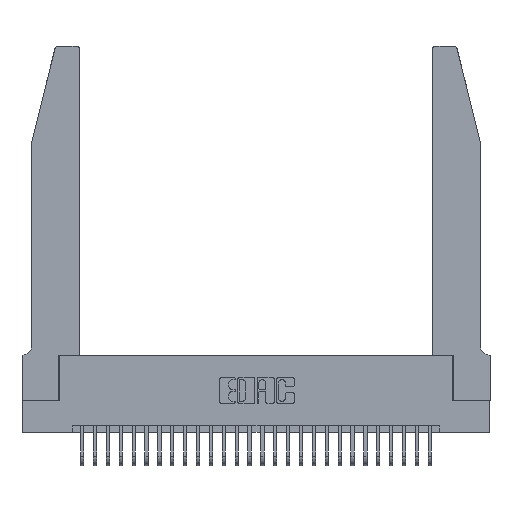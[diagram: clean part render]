
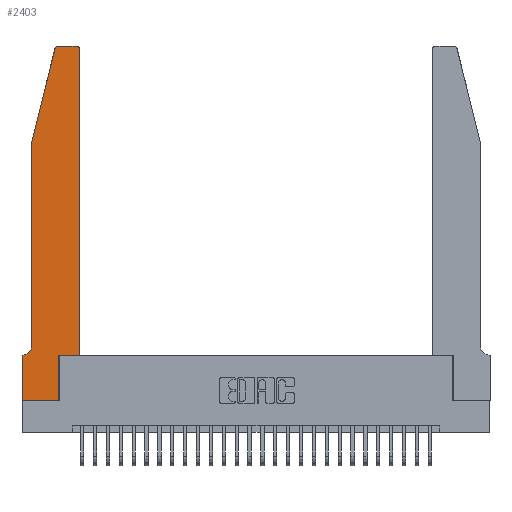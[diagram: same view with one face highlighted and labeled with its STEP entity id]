
A CAD part, top view. The second image highlights one B-rep face of the part: STEP entity #2403.
In plain terms, the highlighted planar face has unit normal (0, 0, 1).
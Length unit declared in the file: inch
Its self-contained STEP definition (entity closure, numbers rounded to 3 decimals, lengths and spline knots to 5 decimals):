
#251 = VECTOR ( 'NONE', #26868, 39.37008 ) ;
#269 = ORIENTED_EDGE ( 'NONE', *, *, #28386, .T. ) ;
#746 = LINE ( 'NONE', #19874, #24188 ) ;
#1655 = ORIENTED_EDGE ( 'NONE', *, *, #4228, .T. ) ;
#1901 = LINE ( 'NONE', #18953, #28568 ) ;
#1916 = CARTESIAN_POINT ( 'NONE',  ( 0., 0.35, 0.37 ) ) ;
#2403 = ADVANCED_FACE ( 'NONE', ( #9724 ), #2414, .T. ) ;
#2414 = PLANE ( 'NONE',  #26581 ) ;
#2914 = DIRECTION ( 'NONE',  ( -1., 0., 0. ) ) ;
#2936 = DIRECTION ( 'NONE',  ( 1., 0., 0. ) ) ;
#3030 = CIRCLE ( 'NONE', #27267, 0.07 ) ;
#3204 = VECTOR ( 'NONE', #20002, 39.37008 ) ;
#3740 = DIRECTION ( 'NONE',  ( 0., -1., 0. ) ) ;
#3985 = VECTOR ( 'NONE', #7193, 39.37008 ) ;
#4228 = EDGE_CURVE ( 'NONE', #15981, #23874, #29718, .T. ) ;
#4891 = LINE ( 'NONE', #24544, #8936 ) ;
#5684 = EDGE_CURVE ( 'NONE', #23874, #6973, #746, .T. ) ;
#6844 = LINE ( 'NONE', #10488, #251 ) ;
#6973 = VERTEX_POINT ( 'NONE', #12463 ) ;
#7193 = DIRECTION ( 'NONE',  ( 0., -1., 0. ) ) ;
#7324 = CARTESIAN_POINT ( 'NONE',  ( 0.4505, 2.72, 0.37 ) ) ;
#7369 = AXIS2_PLACEMENT_3D ( 'NONE', #26047, #12041, #28378 ) ;
#7442 = EDGE_CURVE ( 'NONE', #20556, #12438, #6844, .T. ) ;
#8609 = DIRECTION ( 'NONE',  ( -1., 0., 0. ) ) ;
#8773 = DIRECTION ( 'NONE',  ( 0., 1., 0. ) ) ;
#8936 = VECTOR ( 'NONE', #12594, 39.37008 ) ;
#9724 = FACE_OUTER_BOUND ( 'NONE', #25383, .T. ) ;
#9853 = EDGE_CURVE ( 'NONE', #29273, #20556, #4891, .T. ) ;
#9982 = DIRECTION ( 'NONE',  ( 0., 0., -1. ) ) ;
#10488 = CARTESIAN_POINT ( 'NONE',  ( 0.2865, 0.35, 0.37 ) ) ;
#10535 = CARTESIAN_POINT ( 'NONE',  ( 0.25487, 2.72718, 0.37 ) ) ;
#11016 = VECTOR ( 'NONE', #8609, 39.37008 ) ;
#11150 = ORIENTED_EDGE ( 'NONE', *, *, #7442, .T. ) ;
#12041 = DIRECTION ( 'NONE',  ( 0., 0., 1. ) ) ;
#12438 = VERTEX_POINT ( 'NONE', #26988 ) ;
#12463 = CARTESIAN_POINT ( 'NONE',  ( 0.0755, 2., 0.37 ) ) ;
#12594 = DIRECTION ( 'NONE',  ( 1., 0., 0. ) ) ;
#12718 = ORIENTED_EDGE ( 'NONE', *, *, #13574, .T. ) ;
#13243 = LINE ( 'NONE', #20525, #11016 ) ;
#13470 = LINE ( 'NONE', #15959, #18897 ) ;
#13574 = EDGE_CURVE ( 'NONE', #19607, #29273, #27444, .T. ) ;
#13680 = VERTEX_POINT ( 'NONE', #14955 ) ;
#14571 = DIRECTION ( 'NONE',  ( 1., 0., 0. ) ) ;
#14955 = CARTESIAN_POINT ( 'NONE',  ( 0.0055, 0.35, 0.37 ) ) ;
#15959 = CARTESIAN_POINT ( 'NONE',  ( 0.4505, 0.35, 0.37 ) ) ;
#15981 = VERTEX_POINT ( 'NONE', #26462 ) ;
#16003 = CARTESIAN_POINT ( 'NONE',  ( 0., 0., 0.37 ) ) ;
#16803 = CARTESIAN_POINT ( 'NONE',  ( 0.4505, 0.35, 0.37 ) ) ;
#17055 = VERTEX_POINT ( 'NONE', #28796 ) ;
#17162 = CARTESIAN_POINT ( 'NONE',  ( 0.284, 2.72, 0.37 ) ) ;
#17541 = ORIENTED_EDGE ( 'NONE', *, *, #28021, .T. ) ;
#17554 = ORIENTED_EDGE ( 'NONE', *, *, #30129, .T. ) ;
#17804 = AXIS2_PLACEMENT_3D ( 'NONE', #17162, #21918, #2936 ) ;
#18897 = VECTOR ( 'NONE', #8773, 39.37008 ) ;
#18953 = CARTESIAN_POINT ( 'NONE',  ( 0.4505, 0.35, 0.37 ) ) ;
#19047 = DIRECTION ( 'NONE',  ( 1., 0., 0. ) ) ;
#19137 = CARTESIAN_POINT ( 'NONE',  ( 0., 0., 0.37 ) ) ;
#19276 = ORIENTED_EDGE ( 'NONE', *, *, #9853, .T. ) ;
#19607 = VERTEX_POINT ( 'NONE', #1916 ) ;
#19655 = EDGE_CURVE ( 'NONE', #12438, #20250, #1901, .T. ) ;
#19874 = CARTESIAN_POINT ( 'NONE',  ( 0.0755, 2., 0.37 ) ) ;
#20002 = DIRECTION ( 'NONE',  ( -1., 0., 0. ) ) ;
#20250 = VERTEX_POINT ( 'NONE', #16803 ) ;
#20525 = CARTESIAN_POINT ( 'NONE',  ( 0.2605, 2.75, 0.37 ) ) ;
#20556 = VERTEX_POINT ( 'NONE', #26927 ) ;
#20675 = LINE ( 'NONE', #29260, #24744 ) ;
#20697 = EDGE_CURVE ( 'NONE', #23587, #15981, #13243, .T. ) ;
#21699 = CARTESIAN_POINT ( 'NONE',  ( 0.0055, 0.42, 0.37 ) ) ;
#21786 = DIRECTION ( 'NONE',  ( 0., 0., 1. ) ) ;
#21918 = DIRECTION ( 'NONE',  ( 0., 0., 1. ) ) ;
#22557 = VERTEX_POINT ( 'NONE', #7324 ) ;
#23587 = VERTEX_POINT ( 'NONE', #28223 ) ;
#23874 = VERTEX_POINT ( 'NONE', #10535 ) ;
#24009 = CIRCLE ( 'NONE', #7369, 0.03 ) ;
#24188 = VECTOR ( 'NONE', #26575, 39.37008 ) ;
#24544 = CARTESIAN_POINT ( 'NONE',  ( 0., 0., 0.37 ) ) ;
#24744 = VECTOR ( 'NONE', #3740, 39.37008 ) ;
#25383 = EDGE_LOOP ( 'NONE', ( #28475, #1655, #26660, #27283, #17554, #29741, #12718, #19276, #11150, #30008, #17541, #269 ) ) ;
#25842 = CARTESIAN_POINT ( 'NONE',  ( 0., 0.35, 0.37 ) ) ;
#26047 = CARTESIAN_POINT ( 'NONE',  ( 0.4205, 2.72, 0.37 ) ) ;
#26462 = CARTESIAN_POINT ( 'NONE',  ( 0.284, 2.75, 0.37 ) ) ;
#26575 = DIRECTION ( 'NONE',  ( -0.239, -0.971, 0. ) ) ;
#26581 = AXIS2_PLACEMENT_3D ( 'NONE', #25842, #21786, #14571 ) ;
#26660 = ORIENTED_EDGE ( 'NONE', *, *, #5684, .T. ) ;
#26868 = DIRECTION ( 'NONE',  ( 0., 1., 0. ) ) ;
#26927 = CARTESIAN_POINT ( 'NONE',  ( 0.2865, 0., 0.37 ) ) ;
#26988 = CARTESIAN_POINT ( 'NONE',  ( 0.2865, 0.35, 0.37 ) ) ;
#27236 = CARTESIAN_POINT ( 'NONE',  ( 0.0755, 0.35, 0.37 ) ) ;
#27267 = AXIS2_PLACEMENT_3D ( 'NONE', #21699, #9982, #2914 ) ;
#27283 = ORIENTED_EDGE ( 'NONE', *, *, #28561, .T. ) ;
#27354 = EDGE_CURVE ( 'NONE', #13680, #19607, #30270, .T. ) ;
#27444 = LINE ( 'NONE', #19137, #3985 ) ;
#28021 = EDGE_CURVE ( 'NONE', #20250, #22557, #13470, .T. ) ;
#28223 = CARTESIAN_POINT ( 'NONE',  ( 0.4205, 2.75, 0.37 ) ) ;
#28378 = DIRECTION ( 'NONE',  ( 1., 0., 0. ) ) ;
#28386 = EDGE_CURVE ( 'NONE', #22557, #23587, #24009, .T. ) ;
#28475 = ORIENTED_EDGE ( 'NONE', *, *, #20697, .T. ) ;
#28561 = EDGE_CURVE ( 'NONE', #6973, #17055, #20675, .T. ) ;
#28568 = VECTOR ( 'NONE', #19047, 39.37008 ) ;
#28796 = CARTESIAN_POINT ( 'NONE',  ( 0.0755, 0.42, 0.37 ) ) ;
#29260 = CARTESIAN_POINT ( 'NONE',  ( 0.0755, 2., 0.37 ) ) ;
#29273 = VERTEX_POINT ( 'NONE', #16003 ) ;
#29718 = CIRCLE ( 'NONE', #17804, 0.03 ) ;
#29741 = ORIENTED_EDGE ( 'NONE', *, *, #27354, .T. ) ;
#30008 = ORIENTED_EDGE ( 'NONE', *, *, #19655, .T. ) ;
#30129 = EDGE_CURVE ( 'NONE', #17055, #13680, #3030, .T. ) ;
#30270 = LINE ( 'NONE', #27236, #3204 ) ;
